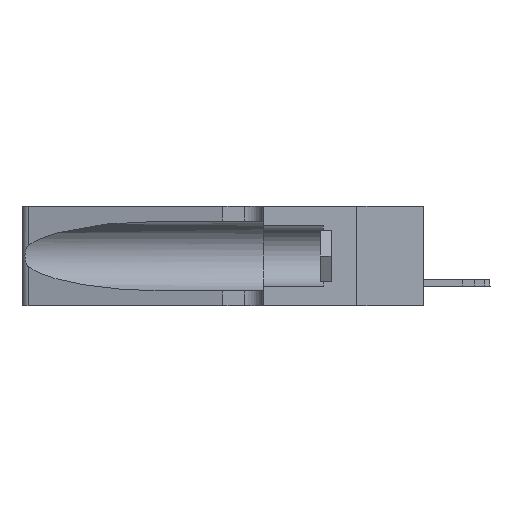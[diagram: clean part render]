
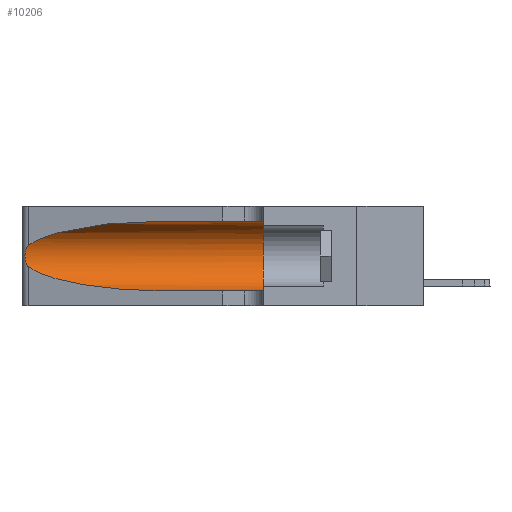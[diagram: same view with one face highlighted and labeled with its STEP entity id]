
A CAD part, left-side view. The second image highlights one B-rep face of the part: STEP entity #10206.
In plain terms, the highlighted cylindrical face has radius 3.308 mm (diameter 6.617 mm), a partial arc.
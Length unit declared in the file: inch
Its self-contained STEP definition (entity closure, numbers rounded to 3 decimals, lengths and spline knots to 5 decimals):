
#112 = CARTESIAN_POINT ( 'NONE',  ( 0.25487, 1.22718, 0.22369 ) ) ;
#473 = DIRECTION ( 'NONE',  ( 0., -1., 0. ) ) ;
#563 = CARTESIAN_POINT ( 'NONE',  ( 0.25487, 1.22718, 0.22369 ) ) ;
#829 = AXIS2_PLACEMENT_3D ( 'NONE', #18977, #3292, #16489 ) ;
#2175 =( BOUNDED_CURVE ( )  B_SPLINE_CURVE ( 3, ( #16544, #20185, #14744, #18610 ),
 .UNSPECIFIED., .F., .F. ) 
 B_SPLINE_CURVE_WITH_KNOTS ( ( 4, 4 ),
 ( 1.5708, 2.84003 ),
 .UNSPECIFIED. ) 
 CURVE ( )  GEOMETRIC_REPRESENTATION_ITEM ( )  RATIONAL_B_SPLINE_CURVE ( ( 1., 0.87, 0.87, 1. ) ) 
 REPRESENTATION_ITEM ( '' )  );
#2637 = CARTESIAN_POINT ( 'NONE',  ( 0.18966, 0.96281, 0.05475 ) ) ;
#3120 = ORIENTED_EDGE ( 'NONE', *, *, #14484, .T. ) ;
#3292 = DIRECTION ( 'NONE',  ( 0., -1., 0. ) ) ;
#3923 = ORIENTED_EDGE ( 'NONE', *, *, #5715, .T. ) ;
#3955 = EDGE_CURVE ( 'NONE', #6506, #15801, #9855, .T. ) ;
#4447 = B_SPLINE_CURVE_WITH_KNOTS ( 'NONE', 3,
 ( #112, #10650, #8638, #4979, #5286, #15871, #7182, #8716, #17510, #7044, #20831, #19382, #8849, #19251 ),
 .UNSPECIFIED., .F., .F.,
 ( 4, 2, 2, 2, 2, 2, 4 ),
 ( 0., 0.00027, 0.00053, 0.00107, 0.0016, 0.00187, 0.00214 ),
 .UNSPECIFIED. ) ;
#4873 = ORIENTED_EDGE ( 'NONE', *, *, #10784, .F. ) ;
#4979 = CARTESIAN_POINT ( 'NONE',  ( 0.25787, 1.23484, 0.2124 ) ) ;
#5286 = CARTESIAN_POINT ( 'NONE',  ( 0.25854, 1.2359, 0.20912 ) ) ;
#5642 = CARTESIAN_POINT ( 'NONE',  ( 0.1305, 1.61858, 0.05475 ) ) ;
#5715 = EDGE_CURVE ( 'NONE', #5789, #9629, #4447, .T. ) ;
#5789 = VERTEX_POINT ( 'NONE', #563 ) ;
#5922 = EDGE_CURVE ( 'NONE', #9629, #6506, #19041, .T. ) ;
#6232 = FACE_OUTER_BOUND ( 'NONE', #16022, .T. ) ;
#6293 = ORIENTED_EDGE ( 'NONE', *, *, #5922, .T. ) ;
#6506 = VERTEX_POINT ( 'NONE', #14986 ) ;
#6881 = ORIENTED_EDGE ( 'NONE', *, *, #10481, .F. ) ;
#7044 = CARTESIAN_POINT ( 'NONE',  ( 0.25856, 1.23593, 0.16098 ) ) ;
#7182 = CARTESIAN_POINT ( 'NONE',  ( 0.26075, 1.23896, 0.19203 ) ) ;
#7317 = CYLINDRICAL_SURFACE ( 'NONE', #829, 0.13025 ) ;
#7888 = AXIS2_PLACEMENT_3D ( 'NONE', #15569, #22546, #8705 ) ;
#8014 = CARTESIAN_POINT ( 'NONE',  ( 0.2373, 1.15595, 0.08982 ) ) ;
#8638 = CARTESIAN_POINT ( 'NONE',  ( 0.25639, 1.23184, 0.21858 ) ) ;
#8705 = DIRECTION ( 'NONE',  ( 0., 0., 1. ) ) ;
#8716 = CARTESIAN_POINT ( 'NONE',  ( 0.26075, 1.23896, 0.178 ) ) ;
#8849 = CARTESIAN_POINT ( 'NONE',  ( 0.25555, 1.22993, 0.14849 ) ) ;
#9427 = CARTESIAN_POINT ( 'NONE',  ( 0.1305, 1.61858, 0.31525 ) ) ;
#9629 = VERTEX_POINT ( 'NONE', #18064 ) ;
#9833 = CARTESIAN_POINT ( 'NONE',  ( 0.1305, 0.72297, 0.05475 ) ) ;
#9855 = LINE ( 'NONE', #5642, #20246 ) ;
#10206 = ADVANCED_FACE ( 'NONE', ( #6232 ), #7317, .F. ) ;
#10481 = EDGE_CURVE ( 'NONE', #17243, #17816, #21742, .T. ) ;
#10650 = CARTESIAN_POINT ( 'NONE',  ( 0.25555, 1.22994, 0.2215 ) ) ;
#10784 = EDGE_CURVE ( 'NONE', #17816, #15801, #17679, .T. ) ;
#11713 = CARTESIAN_POINT ( 'NONE',  ( 0.25487, 1.22718, 0.14631 ) ) ;
#12871 = CARTESIAN_POINT ( 'NONE',  ( 0.1305, 0.72297, 0.31525 ) ) ;
#12986 = VECTOR ( 'NONE', #19977, 39.37008 ) ;
#14484 = EDGE_CURVE ( 'NONE', #17243, #5789, #2175, .T. ) ;
#14744 = CARTESIAN_POINT ( 'NONE',  ( 0.2373, 1.15595, 0.28018 ) ) ;
#14986 = CARTESIAN_POINT ( 'NONE',  ( 0.1305, 0.72297, 0.05475 ) ) ;
#15569 = CARTESIAN_POINT ( 'NONE',  ( 0.1305, 0.35, 0.185 ) ) ;
#15801 = VERTEX_POINT ( 'NONE', #17003 ) ;
#15871 = CARTESIAN_POINT ( 'NONE',  ( 0.26018, 1.23835, 0.19895 ) ) ;
#16022 = EDGE_LOOP ( 'NONE', ( #3120, #3923, #6293, #16916, #4873, #6881 ) ) ;
#16489 = DIRECTION ( 'NONE',  ( 0., 0., -1. ) ) ;
#16544 = CARTESIAN_POINT ( 'NONE',  ( 0.1305, 0.72297, 0.31525 ) ) ;
#16916 = ORIENTED_EDGE ( 'NONE', *, *, #3955, .T. ) ;
#17003 = CARTESIAN_POINT ( 'NONE',  ( 0.1305, 0.35, 0.05475 ) ) ;
#17243 = VERTEX_POINT ( 'NONE', #12871 ) ;
#17510 = CARTESIAN_POINT ( 'NONE',  ( 0.26017, 1.23833, 0.17102 ) ) ;
#17679 = CIRCLE ( 'NONE', #7888, 0.13025 ) ;
#17816 = VERTEX_POINT ( 'NONE', #18416 ) ;
#18064 = CARTESIAN_POINT ( 'NONE',  ( 0.25487, 1.22718, 0.14631 ) ) ;
#18416 = CARTESIAN_POINT ( 'NONE',  ( 0.1305, 0.35, 0.31525 ) ) ;
#18610 = CARTESIAN_POINT ( 'NONE',  ( 0.25487, 1.22718, 0.22369 ) ) ;
#18977 = CARTESIAN_POINT ( 'NONE',  ( 0.1305, 1.61858, 0.185 ) ) ;
#19041 =( BOUNDED_CURVE ( )  B_SPLINE_CURVE ( 3, ( #11713, #8014, #2637, #9833 ),
 .UNSPECIFIED., .F., .F. ) 
 B_SPLINE_CURVE_WITH_KNOTS ( ( 4, 4 ),
 ( 3.44316, 4.71239 ),
 .UNSPECIFIED. ) 
 CURVE ( )  GEOMETRIC_REPRESENTATION_ITEM ( )  RATIONAL_B_SPLINE_CURVE ( ( 1., 0.87, 0.87, 1. ) ) 
 REPRESENTATION_ITEM ( '' )  );
#19251 = CARTESIAN_POINT ( 'NONE',  ( 0.25487, 1.22718, 0.14631 ) ) ;
#19382 = CARTESIAN_POINT ( 'NONE',  ( 0.25639, 1.23186, 0.15144 ) ) ;
#19977 = DIRECTION ( 'NONE',  ( 0., -1., 0. ) ) ;
#20185 = CARTESIAN_POINT ( 'NONE',  ( 0.18966, 0.96281, 0.31525 ) ) ;
#20246 = VECTOR ( 'NONE', #473, 39.37008 ) ;
#20831 = CARTESIAN_POINT ( 'NONE',  ( 0.25789, 1.23486, 0.15765 ) ) ;
#21742 = LINE ( 'NONE', #9427, #12986 ) ;
#22546 = DIRECTION ( 'NONE',  ( 0., 1., 0. ) ) ;
